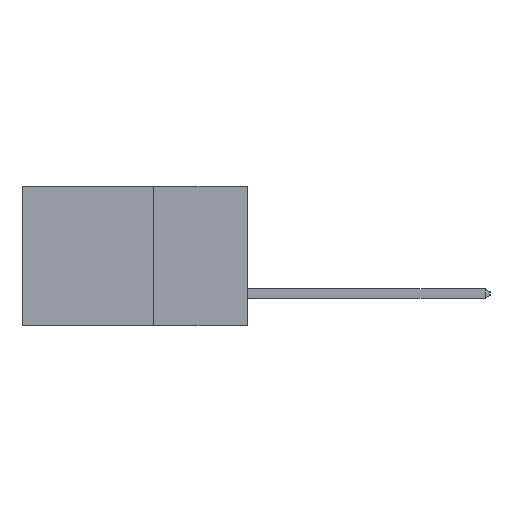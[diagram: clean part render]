
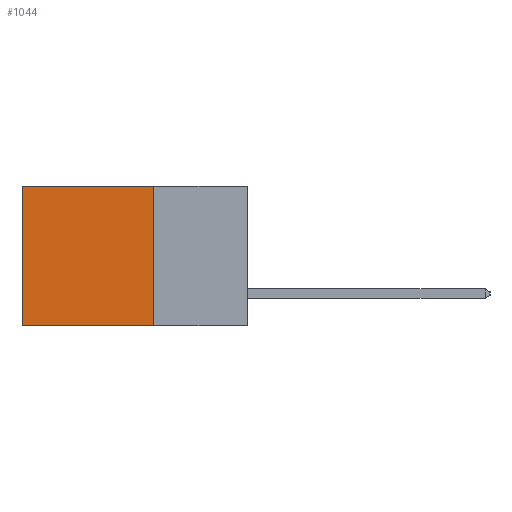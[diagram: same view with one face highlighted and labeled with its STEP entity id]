
A CAD part, left-side view. The second image highlights one B-rep face of the part: STEP entity #1044.
In plain terms, the highlighted planar face has unit normal (-1, 0, 0).
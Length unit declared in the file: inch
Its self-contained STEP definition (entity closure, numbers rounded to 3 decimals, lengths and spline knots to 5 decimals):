
#99 = CARTESIAN_POINT ( 'NONE',  ( 0.298, 0.6, 0. ) ) ;
#657 = VECTOR ( 'NONE', #10519, 39.37008 ) ;
#1044 = ADVANCED_FACE ( 'NONE', ( #2293 ), #7066, .F. ) ;
#1313 = ORIENTED_EDGE ( 'NONE', *, *, #3077, .F. ) ;
#1324 = EDGE_CURVE ( 'NONE', #7807, #3696, #12360, .T. ) ;
#1471 = ORIENTED_EDGE ( 'NONE', *, *, #6477, .F. ) ;
#1610 = LINE ( 'NONE', #6315, #9576 ) ;
#2293 = FACE_OUTER_BOUND ( 'NONE', #10727, .T. ) ;
#2483 = DIRECTION ( 'NONE',  ( 0., 0., -1. ) ) ;
#2789 = VECTOR ( 'NONE', #9886, 39.37008 ) ;
#3077 = EDGE_CURVE ( 'NONE', #9626, #5757, #1610, .T. ) ;
#3238 = AXIS2_PLACEMENT_3D ( 'NONE', #11543, #11142, #3902 ) ;
#3456 = CARTESIAN_POINT ( 'NONE',  ( 0.298, 0.25, 0. ) ) ;
#3621 = ORIENTED_EDGE ( 'NONE', *, *, #1324, .T. ) ;
#3696 = VERTEX_POINT ( 'NONE', #10276 ) ;
#3902 = DIRECTION ( 'NONE',  ( 0., 0., -1. ) ) ;
#4011 = LINE ( 'NONE', #9621, #657 ) ;
#4865 = VECTOR ( 'NONE', #5023, 39.37008 ) ;
#5023 = DIRECTION ( 'NONE',  ( 0., 0., -1. ) ) ;
#5512 = EDGE_CURVE ( 'NONE', #9626, #7807, #10791, .T. ) ;
#5757 = VERTEX_POINT ( 'NONE', #8343 ) ;
#5917 = CARTESIAN_POINT ( 'NONE',  ( 0.298, 0.6, 0. ) ) ;
#6315 = CARTESIAN_POINT ( 'NONE',  ( 0.298, 0.25, 0. ) ) ;
#6477 = EDGE_CURVE ( 'NONE', #5757, #3696, #4011, .T. ) ;
#7066 = PLANE ( 'NONE',  #3238 ) ;
#7807 = VERTEX_POINT ( 'NONE', #99 ) ;
#8343 = CARTESIAN_POINT ( 'NONE',  ( 0.298, 0.25, -0.37 ) ) ;
#8742 = ORIENTED_EDGE ( 'NONE', *, *, #5512, .T. ) ;
#9576 = VECTOR ( 'NONE', #2483, 39.37008 ) ;
#9621 = CARTESIAN_POINT ( 'NONE',  ( 0.298, 0.25, -0.37 ) ) ;
#9626 = VERTEX_POINT ( 'NONE', #3456 ) ;
#9886 = DIRECTION ( 'NONE',  ( 0., 1., 0. ) ) ;
#10276 = CARTESIAN_POINT ( 'NONE',  ( 0.298, 0.6, -0.37 ) ) ;
#10519 = DIRECTION ( 'NONE',  ( 0., 1., 0. ) ) ;
#10727 = EDGE_LOOP ( 'NONE', ( #3621, #1471, #1313, #8742 ) ) ;
#10777 = CARTESIAN_POINT ( 'NONE',  ( 0.298, 0.25, 0. ) ) ;
#10791 = LINE ( 'NONE', #10777, #2789 ) ;
#11142 = DIRECTION ( 'NONE',  ( 1., 0., 0. ) ) ;
#11543 = CARTESIAN_POINT ( 'NONE',  ( 0.298, 0.25, 0. ) ) ;
#12360 = LINE ( 'NONE', #5917, #4865 ) ;
